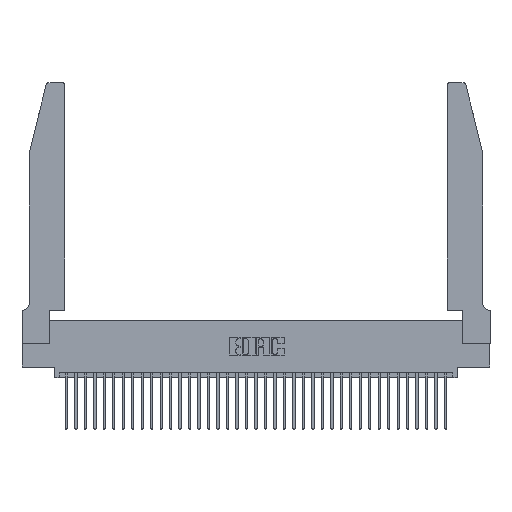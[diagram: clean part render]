
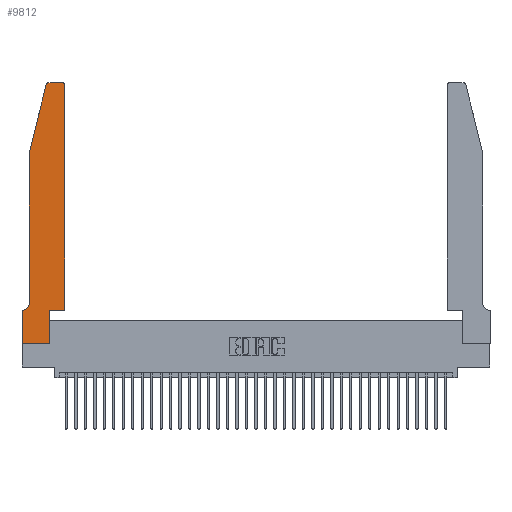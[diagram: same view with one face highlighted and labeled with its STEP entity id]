
A CAD part, top view. The second image highlights one B-rep face of the part: STEP entity #9812.
In plain terms, the highlighted planar face has unit normal (0, 0, 1).
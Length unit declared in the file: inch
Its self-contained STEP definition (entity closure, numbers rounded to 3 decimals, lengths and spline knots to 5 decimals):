
#667 = ORIENTED_EDGE ( 'NONE', *, *, #18832, .T. ) ;
#1386 = CARTESIAN_POINT ( 'NONE',  ( 0., 0.35, 0.37 ) ) ;
#1592 = ORIENTED_EDGE ( 'NONE', *, *, #20113, .T. ) ;
#2347 = CARTESIAN_POINT ( 'NONE',  ( 0.4505, 2.72, 0.37 ) ) ;
#2642 = CARTESIAN_POINT ( 'NONE',  ( 0., 0., 0.37 ) ) ;
#2829 = VERTEX_POINT ( 'NONE', #10845 ) ;
#3229 = VERTEX_POINT ( 'NONE', #32482 ) ;
#3416 = ORIENTED_EDGE ( 'NONE', *, *, #4638, .T. ) ;
#4275 = LINE ( 'NONE', #13974, #11097 ) ;
#4638 = EDGE_CURVE ( 'NONE', #14608, #25742, #19431, .T. ) ;
#5086 = VERTEX_POINT ( 'NONE', #27002 ) ;
#5825 = CIRCLE ( 'NONE', #13343, 0.03 ) ;
#5863 = EDGE_CURVE ( 'NONE', #2829, #5086, #8470, .T. ) ;
#6286 = CIRCLE ( 'NONE', #25680, 0.07 ) ;
#7036 = DIRECTION ( 'NONE',  ( 0., -1., 0. ) ) ;
#7136 = EDGE_CURVE ( 'NONE', #26469, #16915, #4275, .T. ) ;
#7524 = ORIENTED_EDGE ( 'NONE', *, *, #24882, .T. ) ;
#7581 = LINE ( 'NONE', #29985, #37106 ) ;
#8226 = VERTEX_POINT ( 'NONE', #10519 ) ;
#8470 = LINE ( 'NONE', #24337, #30494 ) ;
#8669 = DIRECTION ( 'NONE',  ( 0., 0., 1. ) ) ;
#9658 = LINE ( 'NONE', #16387, #24103 ) ;
#9812 = ADVANCED_FACE ( 'NONE', ( #17975 ), #27415, .T. ) ;
#10373 = AXIS2_PLACEMENT_3D ( 'NONE', #1386, #30276, #13058 ) ;
#10519 = CARTESIAN_POINT ( 'NONE',  ( 0.2865, 0., 0.37 ) ) ;
#10570 = CARTESIAN_POINT ( 'NONE',  ( 0.0055, 0.42, 0.37 ) ) ;
#10797 = CARTESIAN_POINT ( 'NONE',  ( 0.0755, 0.35, 0.37 ) ) ;
#10845 = CARTESIAN_POINT ( 'NONE',  ( 0.0755, 2., 0.37 ) ) ;
#11097 = VECTOR ( 'NONE', #16926, 39.37008 ) ;
#11735 = EDGE_CURVE ( 'NONE', #3229, #2829, #9658, .T. ) ;
#11872 = DIRECTION ( 'NONE',  ( 0., 0., 1. ) ) ;
#12045 = ORIENTED_EDGE ( 'NONE', *, *, #5863, .T. ) ;
#12878 = DIRECTION ( 'NONE',  ( 1., 0., 0. ) ) ;
#13058 = DIRECTION ( 'NONE',  ( 1., 0., 0. ) ) ;
#13343 = AXIS2_PLACEMENT_3D ( 'NONE', #25931, #8669, #28780 ) ;
#13448 = DIRECTION ( 'NONE',  ( -1., 0., 0. ) ) ;
#13681 = DIRECTION ( 'NONE',  ( -1., 0., 0. ) ) ;
#13974 = CARTESIAN_POINT ( 'NONE',  ( 0.4505, 0.35, 0.37 ) ) ;
#14608 = VERTEX_POINT ( 'NONE', #17444 ) ;
#14882 = VERTEX_POINT ( 'NONE', #18430 ) ;
#15571 = CARTESIAN_POINT ( 'NONE',  ( 0.2865, 0.35, 0.37 ) ) ;
#15887 = CARTESIAN_POINT ( 'NONE',  ( 0.4505, 0.35, 0.37 ) ) ;
#16387 = CARTESIAN_POINT ( 'NONE',  ( 0.0755, 2., 0.37 ) ) ;
#16783 = VECTOR ( 'NONE', #21215, 39.37008 ) ;
#16915 = VERTEX_POINT ( 'NONE', #15887 ) ;
#16926 = DIRECTION ( 'NONE',  ( 1., 0., 0. ) ) ;
#17444 = CARTESIAN_POINT ( 'NONE',  ( 0.0055, 0.35, 0.37 ) ) ;
#17975 = FACE_OUTER_BOUND ( 'NONE', #25574, .T. ) ;
#18092 = LINE ( 'NONE', #29070, #32354 ) ;
#18425 = ORIENTED_EDGE ( 'NONE', *, *, #35200, .T. ) ;
#18430 = CARTESIAN_POINT ( 'NONE',  ( 0., 0., 0.37 ) ) ;
#18492 = LINE ( 'NONE', #36863, #27022 ) ;
#18651 = VERTEX_POINT ( 'NONE', #2347 ) ;
#18832 = EDGE_CURVE ( 'NONE', #8226, #26469, #18092, .T. ) ;
#19037 = AXIS2_PLACEMENT_3D ( 'NONE', #29106, #11872, #31920 ) ;
#19431 = LINE ( 'NONE', #10797, #33670 ) ;
#19857 = DIRECTION ( 'NONE',  ( -1., 0., 0. ) ) ;
#20113 = EDGE_CURVE ( 'NONE', #34751, #3229, #21607, .T. ) ;
#21106 = ORIENTED_EDGE ( 'NONE', *, *, #29600, .T. ) ;
#21204 = VECTOR ( 'NONE', #25647, 39.37008 ) ;
#21211 = ORIENTED_EDGE ( 'NONE', *, *, #28701, .T. ) ;
#21215 = DIRECTION ( 'NONE',  ( 0., 1., 0. ) ) ;
#21607 = CIRCLE ( 'NONE', #19037, 0.03 ) ;
#22638 = LINE ( 'NONE', #35379, #16783 ) ;
#24103 = VECTOR ( 'NONE', #25044, 39.37008 ) ;
#24169 = EDGE_CURVE ( 'NONE', #25742, #14882, #29694, .T. ) ;
#24337 = CARTESIAN_POINT ( 'NONE',  ( 0.0755, 2., 0.37 ) ) ;
#24882 = EDGE_CURVE ( 'NONE', #30953, #34751, #18492, .T. ) ;
#25044 = DIRECTION ( 'NONE',  ( -0.239, -0.971, 0. ) ) ;
#25574 = EDGE_LOOP ( 'NONE', ( #7524, #1592, #32220, #12045, #36177, #3416, #31770, #21106, #667, #32230, #18425, #21211 ) ) ;
#25647 = DIRECTION ( 'NONE',  ( 0., -1., 0. ) ) ;
#25680 = AXIS2_PLACEMENT_3D ( 'NONE', #10570, #30659, #13448 ) ;
#25742 = VERTEX_POINT ( 'NONE', #35102 ) ;
#25931 = CARTESIAN_POINT ( 'NONE',  ( 0.4205, 2.72, 0.37 ) ) ;
#26209 = DIRECTION ( 'NONE',  ( 0., 1., 0. ) ) ;
#26469 = VERTEX_POINT ( 'NONE', #15571 ) ;
#27002 = CARTESIAN_POINT ( 'NONE',  ( 0.0755, 0.42, 0.37 ) ) ;
#27022 = VECTOR ( 'NONE', #19857, 39.37008 ) ;
#27415 = PLANE ( 'NONE',  #10373 ) ;
#28486 = EDGE_CURVE ( 'NONE', #5086, #14608, #6286, .T. ) ;
#28701 = EDGE_CURVE ( 'NONE', #18651, #30953, #5825, .T. ) ;
#28780 = DIRECTION ( 'NONE',  ( 1., 0., 0. ) ) ;
#29070 = CARTESIAN_POINT ( 'NONE',  ( 0.2865, 0.35, 0.37 ) ) ;
#29106 = CARTESIAN_POINT ( 'NONE',  ( 0.284, 2.72, 0.37 ) ) ;
#29600 = EDGE_CURVE ( 'NONE', #14882, #8226, #7581, .T. ) ;
#29694 = LINE ( 'NONE', #2642, #21204 ) ;
#29985 = CARTESIAN_POINT ( 'NONE',  ( 0., 0., 0.37 ) ) ;
#30276 = DIRECTION ( 'NONE',  ( 0., 0., 1. ) ) ;
#30494 = VECTOR ( 'NONE', #7036, 39.37008 ) ;
#30659 = DIRECTION ( 'NONE',  ( 0., 0., -1. ) ) ;
#30953 = VERTEX_POINT ( 'NONE', #34789 ) ;
#31770 = ORIENTED_EDGE ( 'NONE', *, *, #24169, .T. ) ;
#31920 = DIRECTION ( 'NONE',  ( 1., 0., 0. ) ) ;
#32220 = ORIENTED_EDGE ( 'NONE', *, *, #11735, .T. ) ;
#32230 = ORIENTED_EDGE ( 'NONE', *, *, #7136, .T. ) ;
#32354 = VECTOR ( 'NONE', #26209, 39.37008 ) ;
#32482 = CARTESIAN_POINT ( 'NONE',  ( 0.25487, 2.72718, 0.37 ) ) ;
#33670 = VECTOR ( 'NONE', #13681, 39.37008 ) ;
#34751 = VERTEX_POINT ( 'NONE', #36385 ) ;
#34789 = CARTESIAN_POINT ( 'NONE',  ( 0.4205, 2.75, 0.37 ) ) ;
#35102 = CARTESIAN_POINT ( 'NONE',  ( 0., 0.35, 0.37 ) ) ;
#35200 = EDGE_CURVE ( 'NONE', #16915, #18651, #22638, .T. ) ;
#35379 = CARTESIAN_POINT ( 'NONE',  ( 0.4505, 0.35, 0.37 ) ) ;
#36177 = ORIENTED_EDGE ( 'NONE', *, *, #28486, .T. ) ;
#36385 = CARTESIAN_POINT ( 'NONE',  ( 0.284, 2.75, 0.37 ) ) ;
#36863 = CARTESIAN_POINT ( 'NONE',  ( 0.2605, 2.75, 0.37 ) ) ;
#37106 = VECTOR ( 'NONE', #12878, 39.37008 ) ;
